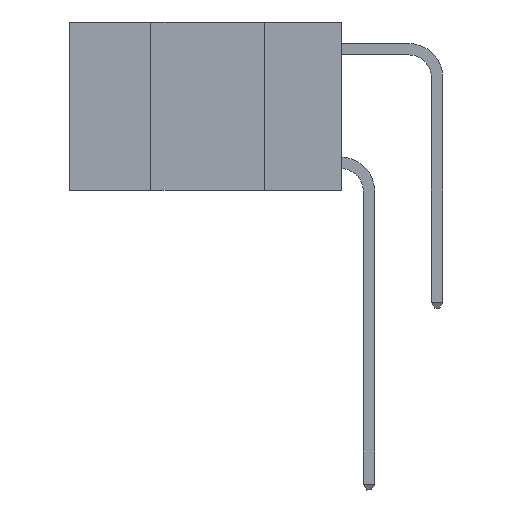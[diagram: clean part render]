
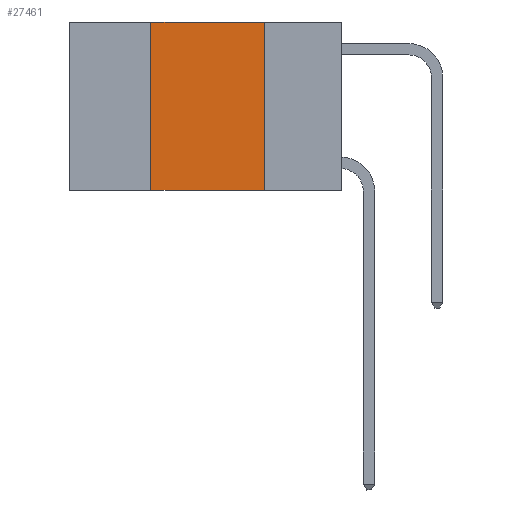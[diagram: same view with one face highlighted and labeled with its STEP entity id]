
A CAD part, left-side view. The second image highlights one B-rep face of the part: STEP entity #27461.
In plain terms, the highlighted planar face has unit normal (-1, 0, 0).
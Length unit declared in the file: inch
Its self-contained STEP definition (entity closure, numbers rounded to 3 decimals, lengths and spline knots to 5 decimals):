
#1176 = DIRECTION ( 'NONE',  ( 0., 0., 1. ) ) ;
#3661 = LINE ( 'NONE', #26823, #32393 ) ;
#3857 = ORIENTED_EDGE ( 'NONE', *, *, #6845, .F. ) ;
#4216 = CARTESIAN_POINT ( 'NONE',  ( 0., 0.6, 0. ) ) ;
#4288 = EDGE_CURVE ( 'NONE', #16009, #28254, #9246, .T. ) ;
#5247 = LINE ( 'NONE', #17590, #17298 ) ;
#6413 = DIRECTION ( 'NONE',  ( 0., 0., -1. ) ) ;
#6845 = EDGE_CURVE ( 'NONE', #7304, #16009, #3661, .T. ) ;
#7304 = VERTEX_POINT ( 'NONE', #26447 ) ;
#7514 = DIRECTION ( 'NONE',  ( 0., -1., 0. ) ) ;
#8219 = CARTESIAN_POINT ( 'NONE',  ( 0., 0.42, 0. ) ) ;
#9246 = LINE ( 'NONE', #32508, #21384 ) ;
#9310 = CARTESIAN_POINT ( 'NONE',  ( 0., 0.17, -0.37 ) ) ;
#9431 = ORIENTED_EDGE ( 'NONE', *, *, #4288, .F. ) ;
#11415 = AXIS2_PLACEMENT_3D ( 'NONE', #4216, #31708, #6413 ) ;
#11420 = PLANE ( 'NONE',  #11415 ) ;
#11776 = CARTESIAN_POINT ( 'NONE',  ( 0., 0.17, 0. ) ) ;
#11928 = ORIENTED_EDGE ( 'NONE', *, *, #28351, .F. ) ;
#12392 = VERTEX_POINT ( 'NONE', #9310 ) ;
#16009 = VERTEX_POINT ( 'NONE', #8219 ) ;
#17298 = VECTOR ( 'NONE', #24902, 39.37008 ) ;
#17590 = CARTESIAN_POINT ( 'NONE',  ( 0., 0.17, 0. ) ) ;
#21384 = VECTOR ( 'NONE', #27672, 39.37008 ) ;
#22503 = LINE ( 'NONE', #32652, #31653 ) ;
#24902 = DIRECTION ( 'NONE',  ( 0., 0., -1. ) ) ;
#24966 = ORIENTED_EDGE ( 'NONE', *, *, #26560, .T. ) ;
#26447 = CARTESIAN_POINT ( 'NONE',  ( 0., 0.42, -0.37 ) ) ;
#26560 = EDGE_CURVE ( 'NONE', #7304, #12392, #22503, .T. ) ;
#26823 = CARTESIAN_POINT ( 'NONE',  ( 0., 0.42, 0. ) ) ;
#27027 = FACE_OUTER_BOUND ( 'NONE', #28340, .T. ) ;
#27461 = ADVANCED_FACE ( 'NONE', ( #27027 ), #11420, .F. ) ;
#27672 = DIRECTION ( 'NONE',  ( 0., -1., 0. ) ) ;
#28254 = VERTEX_POINT ( 'NONE', #11776 ) ;
#28340 = EDGE_LOOP ( 'NONE', ( #11928, #9431, #3857, #24966 ) ) ;
#28351 = EDGE_CURVE ( 'NONE', #28254, #12392, #5247, .T. ) ;
#31653 = VECTOR ( 'NONE', #7514, 39.37008 ) ;
#31708 = DIRECTION ( 'NONE',  ( 1., 0., 0. ) ) ;
#32393 = VECTOR ( 'NONE', #1176, 39.37008 ) ;
#32508 = CARTESIAN_POINT ( 'NONE',  ( 0., 0.6, 0. ) ) ;
#32652 = CARTESIAN_POINT ( 'NONE',  ( 0., 0.6, -0.37 ) ) ;
